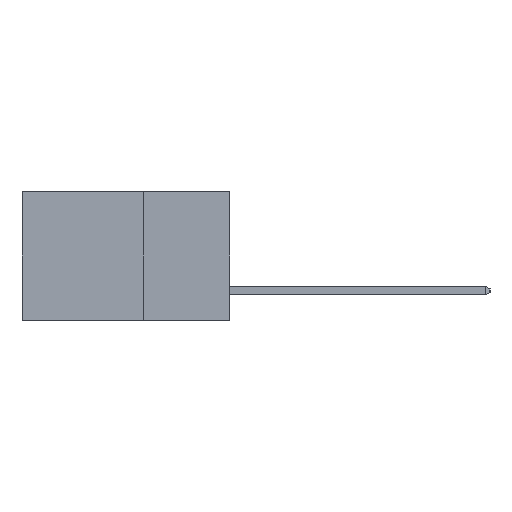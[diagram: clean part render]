
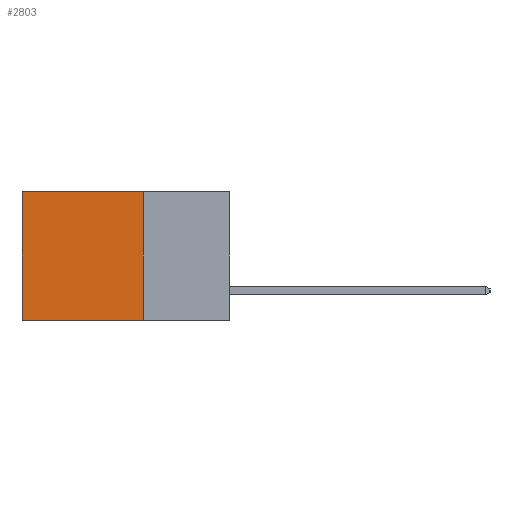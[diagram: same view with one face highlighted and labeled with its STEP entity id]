
A CAD part, left-side view. The second image highlights one B-rep face of the part: STEP entity #2803.
In plain terms, the highlighted planar face has unit normal (-1, 0, 0).
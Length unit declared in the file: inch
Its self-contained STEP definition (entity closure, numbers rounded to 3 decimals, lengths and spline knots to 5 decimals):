
#222 = CARTESIAN_POINT ( 'NONE',  ( 0.298, 0.6, 0. ) ) ;
#756 = VECTOR ( 'NONE', #1961, 39.37008 ) ;
#830 = EDGE_CURVE ( 'NONE', #4247, #8048, #2279, .T. ) ;
#1333 = DIRECTION ( 'NONE',  ( 0., 0., -1. ) ) ;
#1477 = VERTEX_POINT ( 'NONE', #12962 ) ;
#1961 = DIRECTION ( 'NONE',  ( 0., 1., 0. ) ) ;
#2279 = LINE ( 'NONE', #6224, #7602 ) ;
#2374 = ORIENTED_EDGE ( 'NONE', *, *, #6750, .F. ) ;
#2803 = ADVANCED_FACE ( 'NONE', ( #2894 ), #10952, .F. ) ;
#2894 = FACE_OUTER_BOUND ( 'NONE', #7454, .T. ) ;
#3118 = ORIENTED_EDGE ( 'NONE', *, *, #11947, .T. ) ;
#3863 = DIRECTION ( 'NONE',  ( 0., 1., 0. ) ) ;
#4247 = VERTEX_POINT ( 'NONE', #222 ) ;
#4366 = CARTESIAN_POINT ( 'NONE',  ( 0.298, 0.25, 0. ) ) ;
#4940 = ORIENTED_EDGE ( 'NONE', *, *, #830, .T. ) ;
#5145 = CARTESIAN_POINT ( 'NONE',  ( 0.298, 0.25, 0. ) ) ;
#5306 = CARTESIAN_POINT ( 'NONE',  ( 0.298, 0.25, 0. ) ) ;
#5380 = DIRECTION ( 'NONE',  ( 0., 0., -1. ) ) ;
#5548 = LINE ( 'NONE', #11188, #11408 ) ;
#5902 = CARTESIAN_POINT ( 'NONE',  ( 0.298, 0.6, -0.37 ) ) ;
#6224 = CARTESIAN_POINT ( 'NONE',  ( 0.298, 0.6, 0. ) ) ;
#6327 = VERTEX_POINT ( 'NONE', #5306 ) ;
#6379 = ORIENTED_EDGE ( 'NONE', *, *, #9878, .F. ) ;
#6750 = EDGE_CURVE ( 'NONE', #1477, #8048, #5548, .T. ) ;
#7325 = CARTESIAN_POINT ( 'NONE',  ( 0.298, 0.25, 0. ) ) ;
#7342 = DIRECTION ( 'NONE',  ( 1., 0., 0. ) ) ;
#7346 = DIRECTION ( 'NONE',  ( 0., 0., -1. ) ) ;
#7454 = EDGE_LOOP ( 'NONE', ( #4940, #2374, #6379, #3118 ) ) ;
#7602 = VECTOR ( 'NONE', #1333, 39.37008 ) ;
#8048 = VERTEX_POINT ( 'NONE', #5902 ) ;
#9878 = EDGE_CURVE ( 'NONE', #6327, #1477, #13141, .T. ) ;
#9944 = VECTOR ( 'NONE', #5380, 39.37008 ) ;
#10952 = PLANE ( 'NONE',  #13390 ) ;
#11188 = CARTESIAN_POINT ( 'NONE',  ( 0.298, 0.25, -0.37 ) ) ;
#11408 = VECTOR ( 'NONE', #3863, 39.37008 ) ;
#11947 = EDGE_CURVE ( 'NONE', #6327, #4247, #12172, .T. ) ;
#12172 = LINE ( 'NONE', #5145, #756 ) ;
#12962 = CARTESIAN_POINT ( 'NONE',  ( 0.298, 0.25, -0.37 ) ) ;
#13141 = LINE ( 'NONE', #4366, #9944 ) ;
#13390 = AXIS2_PLACEMENT_3D ( 'NONE', #7325, #7342, #7346 ) ;
